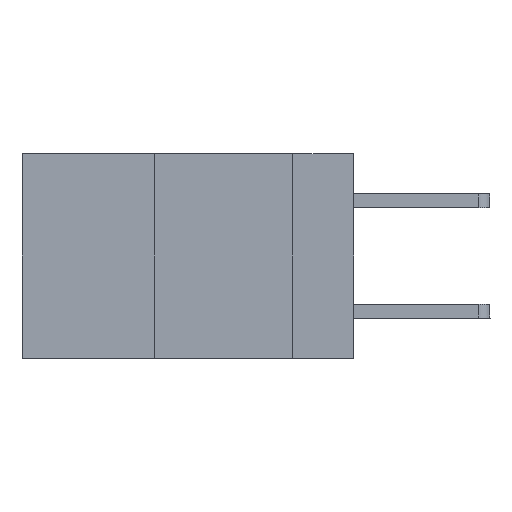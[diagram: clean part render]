
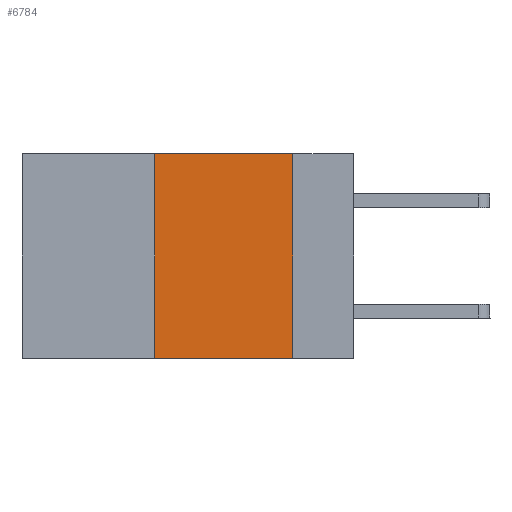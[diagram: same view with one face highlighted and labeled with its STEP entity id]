
A CAD part, left-side view. The second image highlights one B-rep face of the part: STEP entity #6784.
In plain terms, the highlighted planar face has unit normal (-1, 0, 0).
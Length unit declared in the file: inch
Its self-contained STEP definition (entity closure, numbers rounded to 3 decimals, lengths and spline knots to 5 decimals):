
#581 = CARTESIAN_POINT ( 'NONE',  ( 0., 0.6, -0.37 ) ) ;
#819 = DIRECTION ( 'NONE',  ( 0., 0., -1. ) ) ;
#910 = EDGE_CURVE ( 'NONE', #14297, #7909, #5346, .T. ) ;
#983 = ORIENTED_EDGE ( 'NONE', *, *, #13248, .F. ) ;
#1664 = LINE ( 'NONE', #6256, #2256 ) ;
#1697 = LINE ( 'NONE', #3960, #1938 ) ;
#1738 = DIRECTION ( 'NONE',  ( 0., -1., 0. ) ) ;
#1798 = VERTEX_POINT ( 'NONE', #6549 ) ;
#1938 = VECTOR ( 'NONE', #6290, 39.37008 ) ;
#2152 = EDGE_LOOP ( 'NONE', ( #983, #11761, #11893, #7869 ) ) ;
#2256 = VECTOR ( 'NONE', #1738, 39.37008 ) ;
#2939 = VECTOR ( 'NONE', #819, 39.37008 ) ;
#3152 = CARTESIAN_POINT ( 'NONE',  ( 0., 0.11, 0. ) ) ;
#3960 = CARTESIAN_POINT ( 'NONE',  ( 0., 0.36, 0. ) ) ;
#4287 = VERTEX_POINT ( 'NONE', #8922 ) ;
#5346 = LINE ( 'NONE', #581, #13098 ) ;
#6256 = CARTESIAN_POINT ( 'NONE',  ( 0., 0.6, 0. ) ) ;
#6290 = DIRECTION ( 'NONE',  ( 0., 0., 1. ) ) ;
#6549 = CARTESIAN_POINT ( 'NONE',  ( 0., 0.36, 0. ) ) ;
#6744 = FACE_OUTER_BOUND ( 'NONE', #2152, .T. ) ;
#6784 = ADVANCED_FACE ( 'NONE', ( #6744 ), #11248, .F. ) ;
#7327 = EDGE_CURVE ( 'NONE', #14297, #1798, #1697, .T. ) ;
#7460 = AXIS2_PLACEMENT_3D ( 'NONE', #11177, #10347, #8026 ) ;
#7537 = CARTESIAN_POINT ( 'NONE',  ( 0., 0.11, -0.37 ) ) ;
#7869 = ORIENTED_EDGE ( 'NONE', *, *, #910, .T. ) ;
#7909 = VERTEX_POINT ( 'NONE', #7537 ) ;
#8026 = DIRECTION ( 'NONE',  ( 0., 0., -1. ) ) ;
#8922 = CARTESIAN_POINT ( 'NONE',  ( 0., 0.11, 0. ) ) ;
#10347 = DIRECTION ( 'NONE',  ( 1., 0., 0. ) ) ;
#11037 = DIRECTION ( 'NONE',  ( 0., -1., 0. ) ) ;
#11177 = CARTESIAN_POINT ( 'NONE',  ( 0., 0.6, 0. ) ) ;
#11248 = PLANE ( 'NONE',  #7460 ) ;
#11735 = CARTESIAN_POINT ( 'NONE',  ( 0., 0.36, -0.37 ) ) ;
#11761 = ORIENTED_EDGE ( 'NONE', *, *, #14558, .F. ) ;
#11893 = ORIENTED_EDGE ( 'NONE', *, *, #7327, .F. ) ;
#13098 = VECTOR ( 'NONE', #11037, 39.37008 ) ;
#13248 = EDGE_CURVE ( 'NONE', #4287, #7909, #13438, .T. ) ;
#13438 = LINE ( 'NONE', #3152, #2939 ) ;
#14297 = VERTEX_POINT ( 'NONE', #11735 ) ;
#14558 = EDGE_CURVE ( 'NONE', #1798, #4287, #1664, .T. ) ;
